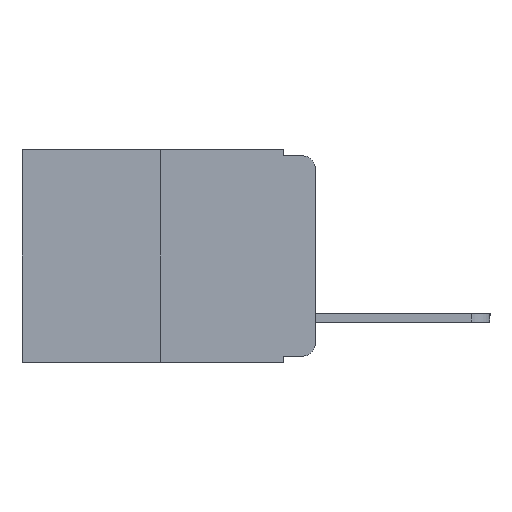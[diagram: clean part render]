
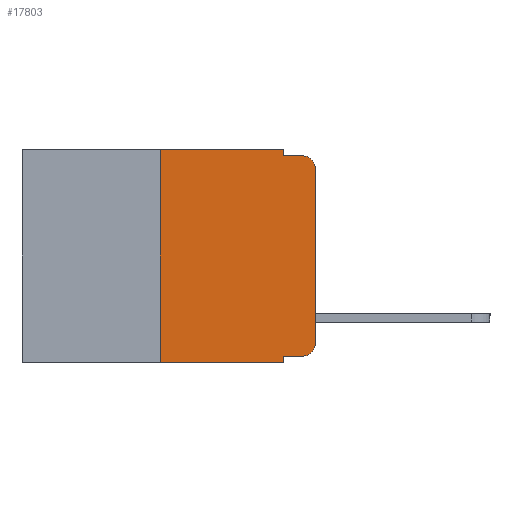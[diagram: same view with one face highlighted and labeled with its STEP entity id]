
A CAD part, left-side view. The second image highlights one B-rep face of the part: STEP entity #17803.
In plain terms, the highlighted planar face has unit normal (-1, 0, 0).
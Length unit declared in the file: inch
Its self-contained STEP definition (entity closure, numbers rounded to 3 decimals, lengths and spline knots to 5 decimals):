
#172 = CARTESIAN_POINT ( 'NONE',  ( 0., 0., 0. ) ) ;
#378 = ORIENTED_EDGE ( 'NONE', *, *, #7300, .T. ) ;
#463 = VECTOR ( 'NONE', #15806, 39.37008 ) ;
#989 = LINE ( 'NONE', #1402, #13158 ) ;
#1402 = CARTESIAN_POINT ( 'NONE',  ( 0., 0.473, -0.343 ) ) ;
#1408 = EDGE_LOOP ( 'NONE', ( #2166, #3659, #9219, #7106, #8518, #7333, #6118, #3469, #378, #6849 ) ) ;
#1422 = VECTOR ( 'NONE', #13681, 39.37008 ) ;
#1767 = VECTOR ( 'NONE', #7717, 39.37008 ) ;
#2125 = CARTESIAN_POINT ( 'NONE',  ( 0., 0.473, 0. ) ) ;
#2166 = ORIENTED_EDGE ( 'NONE', *, *, #4915, .T. ) ;
#2281 = EDGE_CURVE ( 'NONE', #13970, #14359, #15028, .T. ) ;
#2338 = LINE ( 'NONE', #172, #9092 ) ;
#2546 = DIRECTION ( 'NONE',  ( -1., 0., 0. ) ) ;
#2693 = EDGE_CURVE ( 'NONE', #15610, #14359, #8603, .T. ) ;
#3469 = ORIENTED_EDGE ( 'NONE', *, *, #12035, .F. ) ;
#3659 = ORIENTED_EDGE ( 'NONE', *, *, #2281, .T. ) ;
#4087 = VERTEX_POINT ( 'NONE', #18812 ) ;
#4713 = CARTESIAN_POINT ( 'NONE',  ( 0., 0.051, 0. ) ) ;
#4865 = DIRECTION ( 'NONE',  ( 0., 0., 1. ) ) ;
#4915 = EDGE_CURVE ( 'NONE', #7276, #13970, #2338, .T. ) ;
#5303 = DIRECTION ( 'NONE',  ( 1., 0., 0. ) ) ;
#5944 = LINE ( 'NONE', #16442, #1767 ) ;
#6118 = ORIENTED_EDGE ( 'NONE', *, *, #18674, .T. ) ;
#6122 = CARTESIAN_POINT ( 'NONE',  ( 0., 0., -0.313 ) ) ;
#6123 = CARTESIAN_POINT ( 'NONE',  ( 0., 0.02, -0.03 ) ) ;
#6172 = DIRECTION ( 'NONE',  ( 0., -1., 0. ) ) ;
#6243 = CARTESIAN_POINT ( 'NONE',  ( 0., 0.051, -0.343 ) ) ;
#6291 = DIRECTION ( 'NONE',  ( -1., 0., 0. ) ) ;
#6315 = DIRECTION ( 'NONE',  ( 0., 0., -1. ) ) ;
#6849 = ORIENTED_EDGE ( 'NONE', *, *, #11756, .T. ) ;
#7106 = ORIENTED_EDGE ( 'NONE', *, *, #14001, .F. ) ;
#7276 = VERTEX_POINT ( 'NONE', #6122 ) ;
#7300 = EDGE_CURVE ( 'NONE', #14920, #8246, #5944, .T. ) ;
#7333 = ORIENTED_EDGE ( 'NONE', *, *, #11675, .F. ) ;
#7651 = VECTOR ( 'NONE', #12317, 39.37008 ) ;
#7717 = DIRECTION ( 'NONE',  ( 0., -1., 0. ) ) ;
#8246 = VERTEX_POINT ( 'NONE', #16175 ) ;
#8506 = AXIS2_PLACEMENT_3D ( 'NONE', #6123, #6291, #6315 ) ;
#8518 = ORIENTED_EDGE ( 'NONE', *, *, #8728, .F. ) ;
#8603 = LINE ( 'NONE', #11828, #7651 ) ;
#8728 = EDGE_CURVE ( 'NONE', #12878, #11492, #16895, .T. ) ;
#9092 = VECTOR ( 'NONE', #4865, 39.37008 ) ;
#9219 = ORIENTED_EDGE ( 'NONE', *, *, #2693, .F. ) ;
#9278 = FACE_OUTER_BOUND ( 'NONE', #1408, .T. ) ;
#9340 = CARTESIAN_POINT ( 'NONE',  ( 0., 0.051, -0.333 ) ) ;
#9816 = CARTESIAN_POINT ( 'NONE',  ( 0., 0.02, -0.01 ) ) ;
#9875 = AXIS2_PLACEMENT_3D ( 'NONE', #2125, #5303, #15652 ) ;
#10117 = VECTOR ( 'NONE', #14561, 39.37008 ) ;
#11462 = CARTESIAN_POINT ( 'NONE',  ( 0., 0.25, 0. ) ) ;
#11474 = CARTESIAN_POINT ( 'NONE',  ( 0., 0.051, -0.01 ) ) ;
#11492 = VERTEX_POINT ( 'NONE', #18239 ) ;
#11649 = CARTESIAN_POINT ( 'NONE',  ( 0., 0.02, -0.313 ) ) ;
#11675 = EDGE_CURVE ( 'NONE', #4087, #12878, #15609, .T. ) ;
#11756 = EDGE_CURVE ( 'NONE', #8246, #7276, #18017, .T. ) ;
#11828 = CARTESIAN_POINT ( 'NONE',  ( 0., 0.051, -0.01 ) ) ;
#11869 = LINE ( 'NONE', #17747, #15723 ) ;
#12035 = EDGE_CURVE ( 'NONE', #14920, #15981, #13558, .T. ) ;
#12317 = DIRECTION ( 'NONE',  ( 0., -1., 0. ) ) ;
#12878 = VERTEX_POINT ( 'NONE', #16434 ) ;
#13126 = DIRECTION ( 'NONE',  ( 0., 0., -1. ) ) ;
#13158 = VECTOR ( 'NONE', #6172, 39.37008 ) ;
#13558 = LINE ( 'NONE', #4713, #1422 ) ;
#13681 = DIRECTION ( 'NONE',  ( 0., 0., -1. ) ) ;
#13970 = VERTEX_POINT ( 'NONE', #17692 ) ;
#14001 = EDGE_CURVE ( 'NONE', #11492, #15610, #11869, .T. ) ;
#14205 = PLANE ( 'NONE',  #9875 ) ;
#14359 = VERTEX_POINT ( 'NONE', #9816 ) ;
#14561 = DIRECTION ( 'NONE',  ( 0., -1., 0. ) ) ;
#14920 = VERTEX_POINT ( 'NONE', #9340 ) ;
#15028 = CIRCLE ( 'NONE', #8506, 0.02 ) ;
#15068 = AXIS2_PLACEMENT_3D ( 'NONE', #11649, #2546, #13126 ) ;
#15609 = LINE ( 'NONE', #11462, #463 ) ;
#15610 = VERTEX_POINT ( 'NONE', #11474 ) ;
#15652 = DIRECTION ( 'NONE',  ( 0., 0., -1. ) ) ;
#15723 = VECTOR ( 'NONE', #19171, 39.37008 ) ;
#15806 = DIRECTION ( 'NONE',  ( 0., 0., 1. ) ) ;
#15973 = CARTESIAN_POINT ( 'NONE',  ( 0., 0.473, 0. ) ) ;
#15981 = VERTEX_POINT ( 'NONE', #6243 ) ;
#16175 = CARTESIAN_POINT ( 'NONE',  ( 0., 0.02, -0.333 ) ) ;
#16434 = CARTESIAN_POINT ( 'NONE',  ( 0., 0.25, 0. ) ) ;
#16442 = CARTESIAN_POINT ( 'NONE',  ( 0., 0.051, -0.333 ) ) ;
#16895 = LINE ( 'NONE', #15973, #10117 ) ;
#17692 = CARTESIAN_POINT ( 'NONE',  ( 0., 0., -0.03 ) ) ;
#17747 = CARTESIAN_POINT ( 'NONE',  ( 0., 0.051, 0. ) ) ;
#17803 = ADVANCED_FACE ( 'NONE', ( #9278 ), #14205, .F. ) ;
#18017 = CIRCLE ( 'NONE', #15068, 0.02 ) ;
#18239 = CARTESIAN_POINT ( 'NONE',  ( 0., 0.051, 0. ) ) ;
#18674 = EDGE_CURVE ( 'NONE', #4087, #15981, #989, .T. ) ;
#18812 = CARTESIAN_POINT ( 'NONE',  ( 0., 0.25, -0.343 ) ) ;
#19171 = DIRECTION ( 'NONE',  ( 0., 0., -1. ) ) ;
